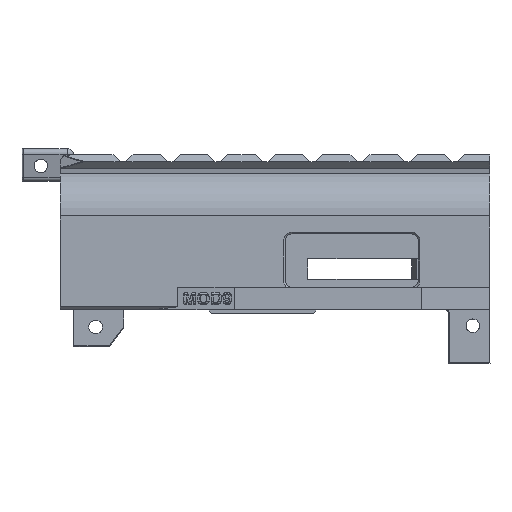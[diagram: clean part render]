
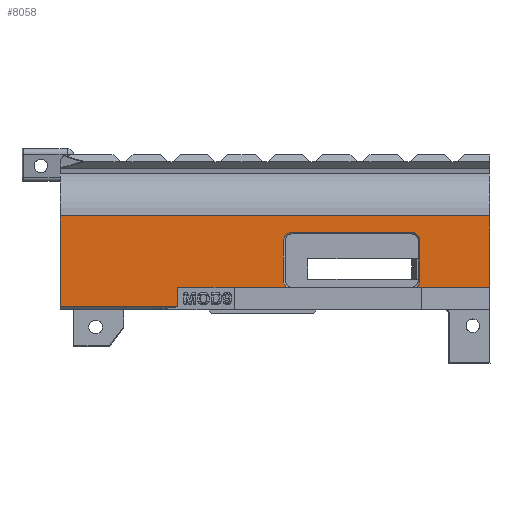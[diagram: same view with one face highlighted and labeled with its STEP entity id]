
A CAD part, top view. The second image highlights one B-rep face of the part: STEP entity #8058.
In plain terms, the highlighted planar face has unit normal (0, 0, 1).
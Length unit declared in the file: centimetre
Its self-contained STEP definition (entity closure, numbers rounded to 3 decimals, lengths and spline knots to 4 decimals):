
#477=FACE_OUTER_BOUND($,#2679,.T.);
#1015=LINE($,#10809,#1821);
#1061=LINE($,#10908,#1867);
#1084=LINE($,#10962,#1890);
#1086=LINE($,#10966,#1892);
#1087=LINE($,#10969,#1893);
#1088=LINE($,#10971,#1894);
#1089=LINE($,#10973,#1895);
#1090=LINE($,#10975,#1896);
#1091=LINE($,#10977,#1897);
#1092=LINE($,#10979,#1898);
#1093=LINE($,#10983,#1899);
#1821=VECTOR($,#9030,3.155);
#1867=VECTOR($,#9092,0.7183);
#1890=VECTOR($,#9135,5.2844);
#1892=VECTOR($,#9139,1.0403);
#1893=VECTOR($,#9142,3.2523);
#1894=VECTOR($,#9143,19.0382);
#1895=VECTOR($,#9144,4.0257);
#1896=VECTOR($,#9145,5.189);
#1897=VECTOR($,#9146,0.8707);
#1898=VECTOR($,#9147,4.846);
#1899=VECTOR($,#9150,1.7606);
#2679=EDGE_LOOP($,(#5456,#5457,#5458,#5459,#5460,#5461,#5462,#5463,#5464,
#5465,#5466,#5467,#5468,#5469,#5470));
#3174=CIRCLE($,#8522,0.38);
#3180=CIRCLE($,#8536,0.38);
#3181=CIRCLE($,#8537,0.38);
#3182=CIRCLE($,#8538,0.38);
#3311=VERTEX_POINT($,#10806);
#3312=VERTEX_POINT($,#10808);
#3353=VERTEX_POINT($,#10897);
#3354=VERTEX_POINT($,#10899);
#3356=VERTEX_POINT($,#10905);
#3378=VERTEX_POINT($,#10961);
#3379=VERTEX_POINT($,#10965);
#3380=VERTEX_POINT($,#10967);
#3381=VERTEX_POINT($,#10970);
#3382=VERTEX_POINT($,#10972);
#3383=VERTEX_POINT($,#10974);
#3384=VERTEX_POINT($,#10976);
#3385=VERTEX_POINT($,#10978);
#3386=VERTEX_POINT($,#10980);
#3387=VERTEX_POINT($,#10982);
#4125=EDGE_CURVE($,#3312,#3311,#1015,.T.);
#4170=EDGE_CURVE($,#3353,#3354,#3174,.T.);
#4174=EDGE_CURVE($,#3356,#3353,#1061,.T.);
#4201=EDGE_CURVE($,#3354,#3378,#1084,.T.);
#4203=EDGE_CURVE($,#3379,#3356,#1086,.T.);
#4204=EDGE_CURVE($,#3380,#3379,#3180,.T.);
#4205=EDGE_CURVE($,#3312,#3380,#1087,.T.);
#4206=EDGE_CURVE($,#3311,#3381,#1088,.T.);
#4207=EDGE_CURVE($,#3381,#3382,#1089,.T.);
#4208=EDGE_CURVE($,#3383,#3382,#1090,.T.);
#4209=EDGE_CURVE($,#3383,#3384,#1091,.T.);
#4210=EDGE_CURVE($,#3385,#3384,#1092,.T.);
#4211=EDGE_CURVE($,#3386,#3385,#3181,.T.);
#4212=EDGE_CURVE($,#3386,#3387,#1093,.T.);
#4213=EDGE_CURVE($,#3378,#3387,#3182,.T.);
#5456=ORIENTED_EDGE($,*,*,#4174,.F.);
#5457=ORIENTED_EDGE($,*,*,#4203,.F.);
#5458=ORIENTED_EDGE($,*,*,#4204,.F.);
#5459=ORIENTED_EDGE($,*,*,#4205,.F.);
#5460=ORIENTED_EDGE($,*,*,#4125,.T.);
#5461=ORIENTED_EDGE($,*,*,#4206,.T.);
#5462=ORIENTED_EDGE($,*,*,#4207,.T.);
#5463=ORIENTED_EDGE($,*,*,#4208,.F.);
#5464=ORIENTED_EDGE($,*,*,#4209,.T.);
#5465=ORIENTED_EDGE($,*,*,#4210,.F.);
#5466=ORIENTED_EDGE($,*,*,#4211,.F.);
#5467=ORIENTED_EDGE($,*,*,#4212,.T.);
#5468=ORIENTED_EDGE($,*,*,#4213,.F.);
#5469=ORIENTED_EDGE($,*,*,#4201,.F.);
#5470=ORIENTED_EDGE($,*,*,#4170,.F.);
#7808=PLANE($,#8535);
#8058=ADVANCED_FACE($,(#477),#7808,.T.);
#8522=AXIS2_PLACEMENT_3D($,#10900,#9084,#9085);
#8535=AXIS2_PLACEMENT_3D($,#10964,#9137,#9138);
#8536=AXIS2_PLACEMENT_3D($,#10968,#9140,#9141);
#8537=AXIS2_PLACEMENT_3D($,#10981,#9148,#9149);
#8538=AXIS2_PLACEMENT_3D($,#10984,#9151,#9152);
#9030=DIRECTION($,(0.,1.,0.));
#9084=DIRECTION('center_axis',(0.,0.,
1.));
#9085=DIRECTION('ref_axis',(0.707,0.707,0.));
#9092=DIRECTION($,(0.,1.,0.));
#9135=DIRECTION($,(-1.,0.,0.));
#9137=DIRECTION('center_axis',(0.,0.,
1.));
#9138=DIRECTION('ref_axis',(1.,0.,0.));
#9139=DIRECTION($,(0.,1.,0.));
#9140=DIRECTION('center_axis',(0.,0.,
1.));
#9141=DIRECTION('ref_axis',(0.707,-0.707,0.));
#9142=DIRECTION($,(-1.,0.,0.));
#9143=DIRECTION($,(-1.,0.,0.));
#9144=DIRECTION($,(0.,-1.,0.));
#9145=DIRECTION($,(-1.,0.,0.));
#9146=DIRECTION($,(0.,1.,0.));
#9147=DIRECTION($,(-1.,0.,0.));
#9148=DIRECTION('center_axis',(0.,0.,
1.));
#9149=DIRECTION('ref_axis',(-0.707,-0.707,0.));
#9150=DIRECTION($,(0.,1.,0.));
#9151=DIRECTION('center_axis',(0.,0.,
1.));
#9152=DIRECTION('ref_axis',(-0.707,0.707,0.));
#10806=CARTESIAN_POINT('',(1.1678,4.7361,2.11));
#10808=CARTESIAN_POINT('',(1.1678,1.5811,2.11));
#10809=CARTESIAN_POINT($,(1.1678,3.994,2.11));
#10897=CARTESIAN_POINT('',(-1.9378,3.6397,2.11));
#10899=CARTESIAN_POINT('',(-2.3178,4.0197,2.11));
#10900=CARTESIAN_POINT('Origin',(-2.3178,3.6397,2.11));
#10905=CARTESIAN_POINT('',(-1.9378,2.9214,2.11));
#10908=CARTESIAN_POINT($,(-1.9378,4.3379,2.11));
#10961=CARTESIAN_POINT('',(-7.6022,4.0197,2.11));
#10962=CARTESIAN_POINT($,(-4.9547,4.0197,2.11));
#10964=CARTESIAN_POINT('Origin',(-2.0072,4.7361,2.11));
#10965=CARTESIAN_POINT('',(-1.9378,1.8811,2.11));
#10966=CARTESIAN_POINT($,(-1.9378,4.3379,2.11));
#10967=CARTESIAN_POINT('',(-2.0846,1.5811,2.11));
#10968=CARTESIAN_POINT('Origin',(-2.3178,1.8811,2.11));
#10969=CARTESIAN_POINT($,(-6.333,1.5811,2.11));
#10970=CARTESIAN_POINT('',(-17.8704,4.7361,2.11));
#10971=CARTESIAN_POINT($,(-2.0072,4.7361,2.11));
#10972=CARTESIAN_POINT('',(-17.8704,0.7104,2.11));
#10973=CARTESIAN_POINT($,(-17.8704,4.7361,2.11));
#10974=CARTESIAN_POINT('',(-12.6814,0.7104,2.11));
#10975=CARTESIAN_POINT($,(-5.4997,0.7104,2.11));
#10976=CARTESIAN_POINT('',(-12.6814,1.5811,2.11));
#10977=CARTESIAN_POINT($,(-12.6814,2.6586,2.11));
#10978=CARTESIAN_POINT('',(-7.8355,1.5811,2.11));
#10979=CARTESIAN_POINT($,(-6.333,1.5811,2.11));
#10980=CARTESIAN_POINT('',(-7.9822,1.8791,2.11));
#10981=CARTESIAN_POINT('Origin',(-7.6022,1.8811,2.11));
#10982=CARTESIAN_POINT('',(-7.9822,3.6397,2.11));
#10983=CARTESIAN_POINT($,(-7.9822,3.7226,2.11));
#10984=CARTESIAN_POINT('Origin',(-7.6022,3.6397,2.11));
